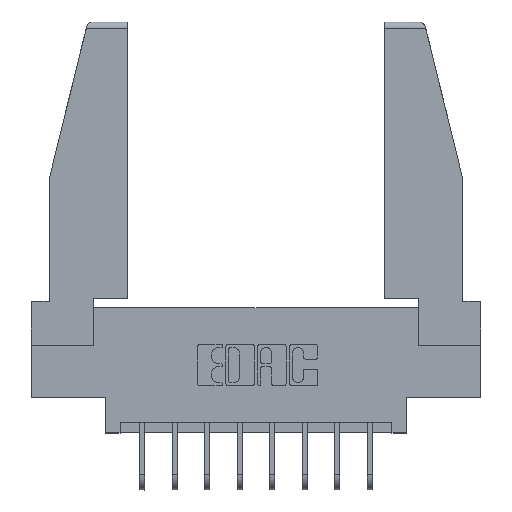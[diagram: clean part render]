
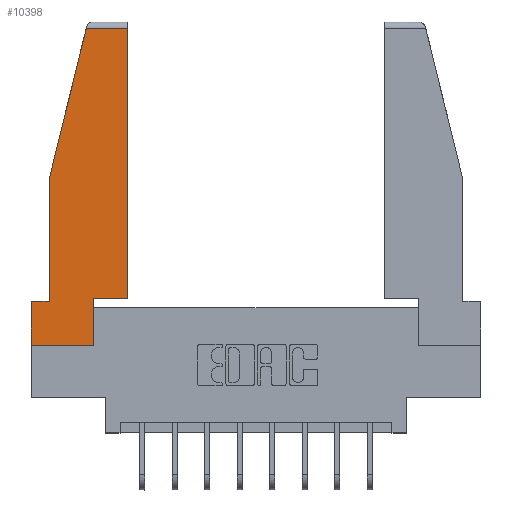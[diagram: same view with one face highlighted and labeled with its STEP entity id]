
A CAD part, top view. The second image highlights one B-rep face of the part: STEP entity #10398.
In plain terms, the highlighted planar face has unit normal (0, 0, 1).
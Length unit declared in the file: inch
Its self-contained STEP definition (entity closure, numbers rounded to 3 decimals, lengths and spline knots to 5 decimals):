
#36 = CARTESIAN_POINT ( 'NONE',  ( 0.297, 0., 0. ) ) ;
#39 = VECTOR ( 'NONE', #1192, 39.37008 ) ;
#460 = EDGE_CURVE ( 'NONE', #4328, #5049, #1478, .T. ) ;
#555 = CARTESIAN_POINT ( 'NONE',  ( 0.086, 0.21, 0. ) ) ;
#771 = VERTEX_POINT ( 'NONE', #10219 ) ;
#1076 = CARTESIAN_POINT ( 'NONE',  ( 0., 0., 0. ) ) ;
#1192 = DIRECTION ( 'NONE',  ( 1., 0., 0. ) ) ;
#1275 = VECTOR ( 'NONE', #2265, 39.37008 ) ;
#1339 = VERTEX_POINT ( 'NONE', #7029 ) ;
#1478 = LINE ( 'NONE', #10664, #6482 ) ;
#1560 = LINE ( 'NONE', #2009, #13018 ) ;
#1562 = ORIENTED_EDGE ( 'NONE', *, *, #10414, .T. ) ;
#1591 = LINE ( 'NONE', #7275, #1275 ) ;
#1713 = CARTESIAN_POINT ( 'NONE',  ( 0.461, 0.223, 0. ) ) ;
#1742 = VECTOR ( 'NONE', #8900, 39.37008 ) ;
#1928 = PLANE ( 'NONE',  #1976 ) ;
#1976 = AXIS2_PLACEMENT_3D ( 'NONE', #8013, #11112, #8969 ) ;
#2009 = CARTESIAN_POINT ( 'NONE',  ( 0., 0.21, 0. ) ) ;
#2084 = EDGE_CURVE ( 'NONE', #771, #6360, #4263, .T. ) ;
#2179 = EDGE_CURVE ( 'NONE', #7524, #5553, #1591, .T. ) ;
#2265 = DIRECTION ( 'NONE',  ( -1., 0., 0. ) ) ;
#2559 = EDGE_CURVE ( 'NONE', #5553, #4328, #12556, .T. ) ;
#3057 = ORIENTED_EDGE ( 'NONE', *, *, #12401, .T. ) ;
#3122 = LINE ( 'NONE', #9811, #8783 ) ;
#3695 = DIRECTION ( 'NONE',  ( 0., 1., 0. ) ) ;
#3710 = ORIENTED_EDGE ( 'NONE', *, *, #7232, .T. ) ;
#4263 = LINE ( 'NONE', #4977, #9296 ) ;
#4328 = VERTEX_POINT ( 'NONE', #4452 ) ;
#4344 = VERTEX_POINT ( 'NONE', #7918 ) ;
#4452 = CARTESIAN_POINT ( 'NONE',  ( 0.086, 0.8, 0. ) ) ;
#4609 = ORIENTED_EDGE ( 'NONE', *, *, #2179, .T. ) ;
#4890 = DIRECTION ( 'NONE',  ( 0., -1., 0. ) ) ;
#4977 = CARTESIAN_POINT ( 'NONE',  ( 0., 0.21, 0. ) ) ;
#5014 = DIRECTION ( 'NONE',  ( -1., 0., 0. ) ) ;
#5049 = VERTEX_POINT ( 'NONE', #555 ) ;
#5065 = ORIENTED_EDGE ( 'NONE', *, *, #460, .T. ) ;
#5455 = VECTOR ( 'NONE', #9675, 39.37008 ) ;
#5553 = VERTEX_POINT ( 'NONE', #9641 ) ;
#5668 = DIRECTION ( 'NONE',  ( 0., -1., 0. ) ) ;
#6270 = CARTESIAN_POINT ( 'NONE',  ( 0.297, 0.223, 0. ) ) ;
#6360 = VERTEX_POINT ( 'NONE', #1076 ) ;
#6482 = VECTOR ( 'NONE', #5668, 39.37008 ) ;
#7029 = CARTESIAN_POINT ( 'NONE',  ( 0.461, 0.223, 0. ) ) ;
#7151 = ORIENTED_EDGE ( 'NONE', *, *, #9556, .T. ) ;
#7172 = ORIENTED_EDGE ( 'NONE', *, *, #2559, .T. ) ;
#7232 = EDGE_CURVE ( 'NONE', #4344, #1339, #11177, .T. ) ;
#7275 = CARTESIAN_POINT ( 'NONE',  ( 0., 1.52, 0. ) ) ;
#7524 = VERTEX_POINT ( 'NONE', #10851 ) ;
#7848 = VECTOR ( 'NONE', #8035, 39.37008 ) ;
#7851 = CARTESIAN_POINT ( 'NONE',  ( 0., 0., 0. ) ) ;
#7918 = CARTESIAN_POINT ( 'NONE',  ( 0.297, 0.223, 0. ) ) ;
#7971 = FACE_OUTER_BOUND ( 'NONE', #10688, .T. ) ;
#8013 = CARTESIAN_POINT ( 'NONE',  ( 0., 0., 0. ) ) ;
#8035 = DIRECTION ( 'NONE',  ( -0.239, -0.971, 0. ) ) ;
#8745 = VERTEX_POINT ( 'NONE', #36 ) ;
#8783 = VECTOR ( 'NONE', #3695, 39.37008 ) ;
#8900 = DIRECTION ( 'NONE',  ( 1., 0., 0. ) ) ;
#8969 = DIRECTION ( 'NONE',  ( 1., 0., 0. ) ) ;
#9217 = ORIENTED_EDGE ( 'NONE', *, *, #2084, .T. ) ;
#9244 = LINE ( 'NONE', #1713, #5455 ) ;
#9296 = VECTOR ( 'NONE', #4890, 39.37008 ) ;
#9556 = EDGE_CURVE ( 'NONE', #8745, #4344, #3122, .T. ) ;
#9641 = CARTESIAN_POINT ( 'NONE',  ( 0.2636, 1.52, 0. ) ) ;
#9675 = DIRECTION ( 'NONE',  ( 0., 1., 0. ) ) ;
#9811 = CARTESIAN_POINT ( 'NONE',  ( 0.297, 0., 0. ) ) ;
#10219 = CARTESIAN_POINT ( 'NONE',  ( 0., 0.21, 0. ) ) ;
#10398 = ADVANCED_FACE ( 'NONE', ( #7971 ), #1928, .T. ) ;
#10414 = EDGE_CURVE ( 'NONE', #5049, #771, #1560, .T. ) ;
#10430 = LINE ( 'NONE', #7851, #1742 ) ;
#10500 = ORIENTED_EDGE ( 'NONE', *, *, #11387, .T. ) ;
#10664 = CARTESIAN_POINT ( 'NONE',  ( 0.086, 0.8, 0. ) ) ;
#10688 = EDGE_LOOP ( 'NONE', ( #3057, #4609, #7172, #5065, #1562, #9217, #10500, #7151, #3710 ) ) ;
#10851 = CARTESIAN_POINT ( 'NONE',  ( 0.461, 1.52, 0. ) ) ;
#11112 = DIRECTION ( 'NONE',  ( 0., 0., 1. ) ) ;
#11177 = LINE ( 'NONE', #6270, #39 ) ;
#11387 = EDGE_CURVE ( 'NONE', #6360, #8745, #10430, .T. ) ;
#12099 = CARTESIAN_POINT ( 'NONE',  ( 0.271, 1.55, 0. ) ) ;
#12401 = EDGE_CURVE ( 'NONE', #1339, #7524, #9244, .T. ) ;
#12556 = LINE ( 'NONE', #12099, #7848 ) ;
#13018 = VECTOR ( 'NONE', #5014, 39.37008 ) ;
